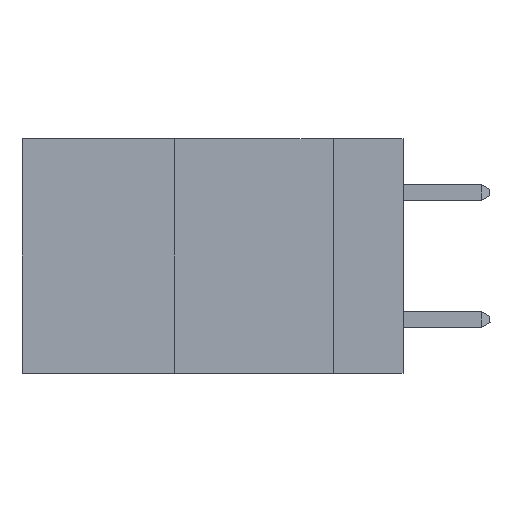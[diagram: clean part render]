
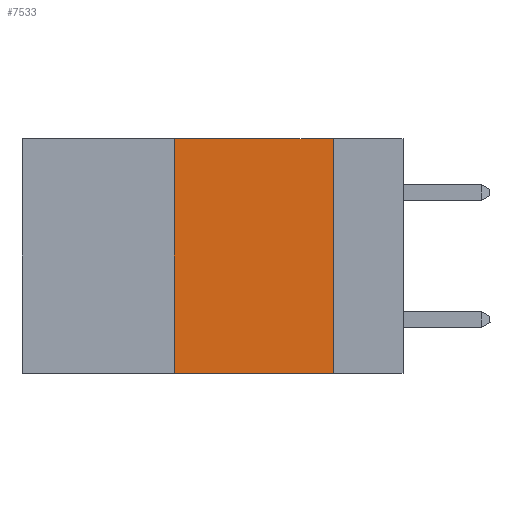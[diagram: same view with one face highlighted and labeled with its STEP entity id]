
A CAD part, left-side view. The second image highlights one B-rep face of the part: STEP entity #7533.
In plain terms, the highlighted planar face has unit normal (-1, 0, 0).
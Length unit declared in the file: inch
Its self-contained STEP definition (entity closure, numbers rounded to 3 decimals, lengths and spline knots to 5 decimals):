
#611 = DIRECTION ( 'NONE',  ( 0., -1., 0. ) ) ;
#758 = ORIENTED_EDGE ( 'NONE', *, *, #6631, .F. ) ;
#1920 = DIRECTION ( 'NONE',  ( 0., -1., 0. ) ) ;
#2606 = EDGE_CURVE ( 'NONE', #7761, #3010, #11166, .T. ) ;
#2707 = ORIENTED_EDGE ( 'NONE', *, *, #8301, .F. ) ;
#3010 = VERTEX_POINT ( 'NONE', #10456 ) ;
#3030 = PLANE ( 'NONE',  #4570 ) ;
#3413 = CARTESIAN_POINT ( 'NONE',  ( 0., 0.36, -0.37 ) ) ;
#4092 = CARTESIAN_POINT ( 'NONE',  ( 0., 0.6, 0. ) ) ;
#4322 = ORIENTED_EDGE ( 'NONE', *, *, #2606, .T. ) ;
#4570 = AXIS2_PLACEMENT_3D ( 'NONE', #4943, #11455, #5866 ) ;
#4869 = VECTOR ( 'NONE', #6919, 39.37008 ) ;
#4943 = CARTESIAN_POINT ( 'NONE',  ( 0., 0.6, 0. ) ) ;
#5095 = CARTESIAN_POINT ( 'NONE',  ( 0., 0.11, 0. ) ) ;
#5866 = DIRECTION ( 'NONE',  ( 0., 0., -1. ) ) ;
#6006 = FACE_OUTER_BOUND ( 'NONE', #6034, .T. ) ;
#6034 = EDGE_LOOP ( 'NONE', ( #2707, #758, #9611, #4322 ) ) ;
#6191 = VECTOR ( 'NONE', #611, 39.37008 ) ;
#6285 = DIRECTION ( 'NONE',  ( 0., 0., 1. ) ) ;
#6627 = VECTOR ( 'NONE', #6285, 39.37008 ) ;
#6631 = EDGE_CURVE ( 'NONE', #11171, #6877, #11223, .T. ) ;
#6877 = VERTEX_POINT ( 'NONE', #9881 ) ;
#6919 = DIRECTION ( 'NONE',  ( 0., 0., -1. ) ) ;
#7209 = CARTESIAN_POINT ( 'NONE',  ( 0., 0.36, 0. ) ) ;
#7533 = ADVANCED_FACE ( 'NONE', ( #6006 ), #3030, .F. ) ;
#7761 = VERTEX_POINT ( 'NONE', #3413 ) ;
#8301 = EDGE_CURVE ( 'NONE', #6877, #3010, #12245, .T. ) ;
#9166 = CARTESIAN_POINT ( 'NONE',  ( 0., 0.6, -0.37 ) ) ;
#9611 = ORIENTED_EDGE ( 'NONE', *, *, #12249, .F. ) ;
#9881 = CARTESIAN_POINT ( 'NONE',  ( 0., 0.11, 0. ) ) ;
#10456 = CARTESIAN_POINT ( 'NONE',  ( 0., 0.11, -0.37 ) ) ;
#11166 = LINE ( 'NONE', #9166, #6191 ) ;
#11171 = VERTEX_POINT ( 'NONE', #11218 ) ;
#11218 = CARTESIAN_POINT ( 'NONE',  ( 0., 0.36, 0. ) ) ;
#11223 = LINE ( 'NONE', #4092, #11504 ) ;
#11455 = DIRECTION ( 'NONE',  ( 1., 0., 0. ) ) ;
#11504 = VECTOR ( 'NONE', #1920, 39.37008 ) ;
#11592 = LINE ( 'NONE', #7209, #6627 ) ;
#12245 = LINE ( 'NONE', #5095, #4869 ) ;
#12249 = EDGE_CURVE ( 'NONE', #7761, #11171, #11592, .T. ) ;
